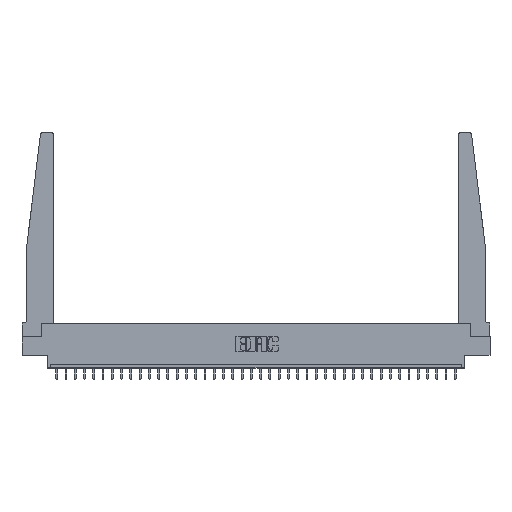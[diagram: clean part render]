
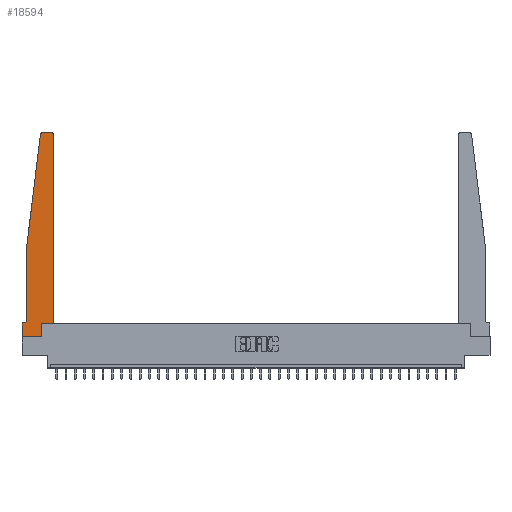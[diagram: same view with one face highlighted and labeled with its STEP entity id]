
A CAD part, top view. The second image highlights one B-rep face of the part: STEP entity #18594.
In plain terms, the highlighted planar face has unit normal (0, 0, 1).
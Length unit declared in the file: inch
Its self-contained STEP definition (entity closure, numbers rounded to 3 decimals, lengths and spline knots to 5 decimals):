
#311 = VECTOR ( 'NONE', #21992, 39.37008 ) ;
#472 = CARTESIAN_POINT ( 'NONE',  ( 0.2605, 0., 0.37 ) ) ;
#585 = DIRECTION ( 'NONE',  ( 0., 1., 0. ) ) ;
#907 = VERTEX_POINT ( 'NONE', #13213 ) ;
#1058 = DIRECTION ( 'NONE',  ( 1., 0., 0. ) ) ;
#1421 = ORIENTED_EDGE ( 'NONE', *, *, #26807, .T. ) ;
#2171 = DIRECTION ( 'NONE',  ( 1., 0., 0. ) ) ;
#2744 = CARTESIAN_POINT ( 'NONE',  ( 0.065, 1.25, 0.37 ) ) ;
#2875 = CARTESIAN_POINT ( 'NONE',  ( 0.065, 0.1875, 0.37 ) ) ;
#2983 = VERTEX_POINT ( 'NONE', #23278 ) ;
#3253 = DIRECTION ( 'NONE',  ( 0., -1., 0. ) ) ;
#3303 = VECTOR ( 'NONE', #3253, 39.37008 ) ;
#3438 = VERTEX_POINT ( 'NONE', #30295 ) ;
#3859 = AXIS2_PLACEMENT_3D ( 'NONE', #11916, #26876, #2171 ) ;
#4031 = CARTESIAN_POINT ( 'NONE',  ( 0.395, 2.75, 0.37 ) ) ;
#4740 = ORIENTED_EDGE ( 'NONE', *, *, #16270, .T. ) ;
#4939 = EDGE_CURVE ( 'NONE', #2983, #3438, #16734, .T. ) ;
#4987 = CARTESIAN_POINT ( 'NONE',  ( 0.425, 2.72, 0.37 ) ) ;
#5118 = VECTOR ( 'NONE', #21781, 39.37008 ) ;
#5326 = EDGE_CURVE ( 'NONE', #19943, #6169, #25960, .T. ) ;
#5405 = ORIENTED_EDGE ( 'NONE', *, *, #4939, .T. ) ;
#5849 = PLANE ( 'NONE',  #17374 ) ;
#5852 = EDGE_LOOP ( 'NONE', ( #21697, #19464, #20514, #1421, #5935, #20616, #5405, #22845, #6426, #19053, #28889, #4740 ) ) ;
#5857 = LINE ( 'NONE', #31701, #27434 ) ;
#5935 = ORIENTED_EDGE ( 'NONE', *, *, #17813, .T. ) ;
#6169 = VERTEX_POINT ( 'NONE', #23425 ) ;
#6300 = DIRECTION ( 'NONE',  ( -1., 0., 0. ) ) ;
#6426 = ORIENTED_EDGE ( 'NONE', *, *, #14483, .T. ) ;
#6689 = CARTESIAN_POINT ( 'NONE',  ( 0.065, 1.25, 0.37 ) ) ;
#7158 = DIRECTION ( 'NONE',  ( 1., 0., 0. ) ) ;
#7317 = VERTEX_POINT ( 'NONE', #4031 ) ;
#7534 = DIRECTION ( 'NONE',  ( 0., -1., 0. ) ) ;
#8442 = CARTESIAN_POINT ( 'NONE',  ( 0., 0.1875, 0.37 ) ) ;
#10131 = LINE ( 'NONE', #6689, #5118 ) ;
#10962 = VECTOR ( 'NONE', #585, 39.37008 ) ;
#11916 = CARTESIAN_POINT ( 'NONE',  ( 0.27653, 2.72, 0.37 ) ) ;
#12075 = EDGE_CURVE ( 'NONE', #3438, #12428, #5857, .T. ) ;
#12195 = LINE ( 'NONE', #25463, #3303 ) ;
#12239 = VECTOR ( 'NONE', #17432, 39.37008 ) ;
#12428 = VERTEX_POINT ( 'NONE', #472 ) ;
#13000 = DIRECTION ( 'NONE',  ( 0., 0., 1. ) ) ;
#13213 = CARTESIAN_POINT ( 'NONE',  ( 0.065, 0.2375, 0.37 ) ) ;
#13711 = VECTOR ( 'NONE', #20409, 39.37008 ) ;
#13828 = VERTEX_POINT ( 'NONE', #29251 ) ;
#14483 = EDGE_CURVE ( 'NONE', #12428, #13828, #18462, .T. ) ;
#15672 = CARTESIAN_POINT ( 'NONE',  ( 0.395, 2.72, 0.37 ) ) ;
#16060 = CARTESIAN_POINT ( 'NONE',  ( 0.425, 0.18, 0.37 ) ) ;
#16270 = EDGE_CURVE ( 'NONE', #27318, #7317, #22162, .T. ) ;
#16734 = LINE ( 'NONE', #17378, #21388 ) ;
#17374 = AXIS2_PLACEMENT_3D ( 'NONE', #8442, #20561, #30619 ) ;
#17378 = CARTESIAN_POINT ( 'NONE',  ( 0., 0., 0.37 ) ) ;
#17432 = DIRECTION ( 'NONE',  ( -1., 0., 0. ) ) ;
#17645 = EDGE_CURVE ( 'NONE', #13828, #22501, #31546, .T. ) ;
#17813 = EDGE_CURVE ( 'NONE', #907, #18938, #23449, .T. ) ;
#18380 = EDGE_CURVE ( 'NONE', #7317, #19943, #29185, .T. ) ;
#18462 = LINE ( 'NONE', #28993, #30741 ) ;
#18594 = ADVANCED_FACE ( 'NONE', ( #28771 ), #5849, .T. ) ;
#18910 = DIRECTION ( 'NONE',  ( 0., 1., 0. ) ) ;
#18938 = VERTEX_POINT ( 'NONE', #22204 ) ;
#19053 = ORIENTED_EDGE ( 'NONE', *, *, #17645, .T. ) ;
#19464 = ORIENTED_EDGE ( 'NONE', *, *, #5326, .T. ) ;
#19850 = CARTESIAN_POINT ( 'NONE',  ( 0.27653, 2.75, 0.37 ) ) ;
#19943 = VERTEX_POINT ( 'NONE', #19850 ) ;
#20253 = LINE ( 'NONE', #30013, #10962 ) ;
#20409 = DIRECTION ( 'NONE',  ( -1., 0., 0. ) ) ;
#20514 = ORIENTED_EDGE ( 'NONE', *, *, #29496, .T. ) ;
#20561 = DIRECTION ( 'NONE',  ( 0., 0., 1. ) ) ;
#20616 = ORIENTED_EDGE ( 'NONE', *, *, #27430, .T. ) ;
#20911 = EDGE_CURVE ( 'NONE', #22501, #27318, #20253, .T. ) ;
#21247 = AXIS2_PLACEMENT_3D ( 'NONE', #15672, #13000, #1058 ) ;
#21325 = VERTEX_POINT ( 'NONE', #2744 ) ;
#21388 = VECTOR ( 'NONE', #7534, 39.37008 ) ;
#21697 = ORIENTED_EDGE ( 'NONE', *, *, #18380, .T. ) ;
#21781 = DIRECTION ( 'NONE',  ( -0.122, -0.992, 0. ) ) ;
#21992 = DIRECTION ( 'NONE',  ( 1., 0., 0. ) ) ;
#22162 = CIRCLE ( 'NONE', #21247, 0.03 ) ;
#22204 = CARTESIAN_POINT ( 'NONE',  ( 0.015, 0.1875, 0.37 ) ) ;
#22501 = VERTEX_POINT ( 'NONE', #16060 ) ;
#22845 = ORIENTED_EDGE ( 'NONE', *, *, #12075, .T. ) ;
#23278 = CARTESIAN_POINT ( 'NONE',  ( 0., 0.1875, 0.37 ) ) ;
#23425 = CARTESIAN_POINT ( 'NONE',  ( 0.24675, 2.72367, 0.37 ) ) ;
#23449 = CIRCLE ( 'NONE', #28468, 0.05 ) ;
#24804 = CARTESIAN_POINT ( 'NONE',  ( 0.25, 2.75, 0.37 ) ) ;
#25463 = CARTESIAN_POINT ( 'NONE',  ( 0.065, 1.25, 0.37 ) ) ;
#25960 = CIRCLE ( 'NONE', #3859, 0.03 ) ;
#26807 = EDGE_CURVE ( 'NONE', #21325, #907, #12195, .T. ) ;
#26876 = DIRECTION ( 'NONE',  ( 0., 0., 1. ) ) ;
#27318 = VERTEX_POINT ( 'NONE', #4987 ) ;
#27430 = EDGE_CURVE ( 'NONE', #18938, #2983, #30642, .T. ) ;
#27434 = VECTOR ( 'NONE', #7158, 39.37008 ) ;
#28468 = AXIS2_PLACEMENT_3D ( 'NONE', #30952, #30750, #6300 ) ;
#28771 = FACE_OUTER_BOUND ( 'NONE', #5852, .T. ) ;
#28889 = ORIENTED_EDGE ( 'NONE', *, *, #20911, .T. ) ;
#28993 = CARTESIAN_POINT ( 'NONE',  ( 0.2605, 0.18, 0.37 ) ) ;
#29185 = LINE ( 'NONE', #24804, #12239 ) ;
#29251 = CARTESIAN_POINT ( 'NONE',  ( 0.2605, 0.18, 0.37 ) ) ;
#29496 = EDGE_CURVE ( 'NONE', #6169, #21325, #10131, .T. ) ;
#30013 = CARTESIAN_POINT ( 'NONE',  ( 0.425, 0.18, 0.37 ) ) ;
#30295 = CARTESIAN_POINT ( 'NONE',  ( 0., 0., 0.37 ) ) ;
#30619 = DIRECTION ( 'NONE',  ( 1., 0., 0. ) ) ;
#30642 = LINE ( 'NONE', #2875, #13711 ) ;
#30741 = VECTOR ( 'NONE', #18910, 39.37008 ) ;
#30750 = DIRECTION ( 'NONE',  ( 0., 0., -1. ) ) ;
#30952 = CARTESIAN_POINT ( 'NONE',  ( 0.015, 0.2375, 0.37 ) ) ;
#31546 = LINE ( 'NONE', #31758, #311 ) ;
#31701 = CARTESIAN_POINT ( 'NONE',  ( 0., 0., 0.37 ) ) ;
#31758 = CARTESIAN_POINT ( 'NONE',  ( 0.425, 0.18, 0.37 ) ) ;
